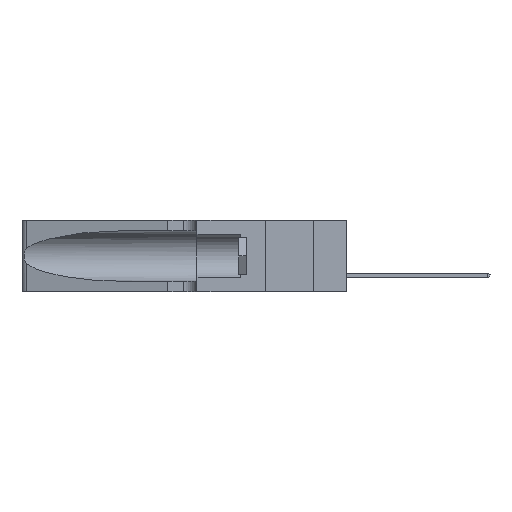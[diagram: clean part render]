
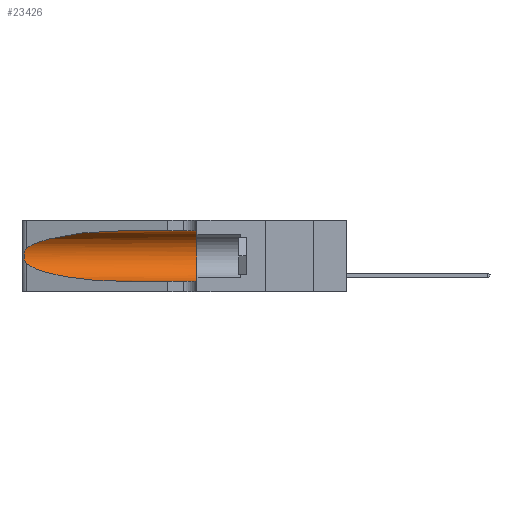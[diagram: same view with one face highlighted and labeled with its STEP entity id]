
A CAD part, left-side view. The second image highlights one B-rep face of the part: STEP entity #23426.
In plain terms, the highlighted cylindrical face has radius 3.308 mm (diameter 6.617 mm), a partial arc.
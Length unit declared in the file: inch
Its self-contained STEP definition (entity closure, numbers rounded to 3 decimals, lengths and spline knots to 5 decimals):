
#1093 = CARTESIAN_POINT ( 'NONE',  ( 0.25639, 1.23184, 0.21858 ) ) ;
#1326 = ORIENTED_EDGE ( 'NONE', *, *, #24503, .F. ) ;
#1364 = CARTESIAN_POINT ( 'NONE',  ( 0.25555, 1.22993, 0.14849 ) ) ;
#1532 = CARTESIAN_POINT ( 'NONE',  ( 0.25487, 1.22718, 0.14631 ) ) ;
#1746 = VECTOR ( 'NONE', #34111, 39.37008 ) ;
#1956 = CARTESIAN_POINT ( 'NONE',  ( 0.18966, 0.96281, 0.05475 ) ) ;
#2602 = CARTESIAN_POINT ( 'NONE',  ( 0.25487, 1.22718, 0.22369 ) ) ;
#3010 = ORIENTED_EDGE ( 'NONE', *, *, #10201, .T. ) ;
#3839 = CARTESIAN_POINT ( 'NONE',  ( 0.25854, 1.2359, 0.20912 ) ) ;
#4182 = ORIENTED_EDGE ( 'NONE', *, *, #31399, .T. ) ;
#5484 = CARTESIAN_POINT ( 'NONE',  ( 0.1305, 0.72297, 0.05475 ) ) ;
#6880 = VERTEX_POINT ( 'NONE', #2602 ) ;
#6938 = ORIENTED_EDGE ( 'NONE', *, *, #25981, .T. ) ;
#6971 = CARTESIAN_POINT ( 'NONE',  ( 0.25789, 1.23486, 0.15765 ) ) ;
#7225 = CARTESIAN_POINT ( 'NONE',  ( 0.26075, 1.23896, 0.178 ) ) ;
#7509 = CARTESIAN_POINT ( 'NONE',  ( 0.1305, 1.61858, 0.185 ) ) ;
#8089 = CIRCLE ( 'NONE', #18900, 0.13025 ) ;
#9688 = CARTESIAN_POINT ( 'NONE',  ( 0.18966, 0.96281, 0.31525 ) ) ;
#10201 = EDGE_CURVE ( 'NONE', #22672, #24491, #25761, .T. ) ;
#10582 = DIRECTION ( 'NONE',  ( 0., -1., 0. ) ) ;
#10909 = CARTESIAN_POINT ( 'NONE',  ( 0.1305, 1.61858, 0.31525 ) ) ;
#12730 = CARTESIAN_POINT ( 'NONE',  ( 0.25856, 1.23593, 0.16098 ) ) ;
#12855 = CARTESIAN_POINT ( 'NONE',  ( 0.25487, 1.22718, 0.22369 ) ) ;
#13667 = DIRECTION ( 'NONE',  ( 0., 0., -1. ) ) ;
#14142 = FACE_OUTER_BOUND ( 'NONE', #27985, .T. ) ;
#15174 = CARTESIAN_POINT ( 'NONE',  ( 0.1305, 1.61858, 0.05475 ) ) ;
#15596 = DIRECTION ( 'NONE',  ( 0., 1., 0. ) ) ;
#15795 = CARTESIAN_POINT ( 'NONE',  ( 0.25487, 1.22718, 0.14631 ) ) ;
#15982 = DIRECTION ( 'NONE',  ( 0., 0., 1. ) ) ;
#16223 = ORIENTED_EDGE ( 'NONE', *, *, #31005, .T. ) ;
#17712 = CARTESIAN_POINT ( 'NONE',  ( 0.1305, 0.72297, 0.05475 ) ) ;
#17826 = EDGE_CURVE ( 'NONE', #21288, #20216, #31760, .T. ) ;
#18103 = DIRECTION ( 'NONE',  ( 0., -1., 0. ) ) ;
#18900 = AXIS2_PLACEMENT_3D ( 'NONE', #33681, #15596, #15982 ) ;
#19483 = ORIENTED_EDGE ( 'NONE', *, *, #17826, .F. ) ;
#20050 = CARTESIAN_POINT ( 'NONE',  ( 0.1305, 0.35, 0.31525 ) ) ;
#20216 = VERTEX_POINT ( 'NONE', #20050 ) ;
#21013 = CARTESIAN_POINT ( 'NONE',  ( 0.1305, 0.72297, 0.31525 ) ) ;
#21127 = CARTESIAN_POINT ( 'NONE',  ( 0.25487, 1.22718, 0.22369 ) ) ;
#21288 = VERTEX_POINT ( 'NONE', #33509 ) ;
#22672 = VERTEX_POINT ( 'NONE', #17712 ) ;
#22736 = CARTESIAN_POINT ( 'NONE',  ( 0.2373, 1.15595, 0.08982 ) ) ;
#22876 = VERTEX_POINT ( 'NONE', #1532 ) ;
#23426 = ADVANCED_FACE ( 'NONE', ( #14142 ), #28499, .F. ) ;
#24485 = CARTESIAN_POINT ( 'NONE',  ( 0.25555, 1.22994, 0.2215 ) ) ;
#24491 = VERTEX_POINT ( 'NONE', #33408 ) ;
#24503 = EDGE_CURVE ( 'NONE', #20216, #24491, #8089, .T. ) ;
#25761 = LINE ( 'NONE', #15174, #37788 ) ;
#25981 = EDGE_CURVE ( 'NONE', #21288, #6880, #32494, .T. ) ;
#26233 = AXIS2_PLACEMENT_3D ( 'NONE', #7509, #10582, #13667 ) ;
#27466 = CARTESIAN_POINT ( 'NONE',  ( 0.25639, 1.23186, 0.15144 ) ) ;
#27984 = CARTESIAN_POINT ( 'NONE',  ( 0.25787, 1.23484, 0.2124 ) ) ;
#27985 = EDGE_LOOP ( 'NONE', ( #6938, #4182, #16223, #3010, #1326, #19483 ) ) ;
#28499 = CYLINDRICAL_SURFACE ( 'NONE', #26233, 0.13025 ) ;
#29802 = CARTESIAN_POINT ( 'NONE',  ( 0.2373, 1.15595, 0.28018 ) ) ;
#31005 = EDGE_CURVE ( 'NONE', #22876, #22672, #34169, .T. ) ;
#31399 = EDGE_CURVE ( 'NONE', #6880, #22876, #37011, .T. ) ;
#31760 = LINE ( 'NONE', #10909, #1746 ) ;
#32494 =( BOUNDED_CURVE ( )  B_SPLINE_CURVE ( 3, ( #21013, #9688, #29802, #21127 ),
 .UNSPECIFIED., .F., .T. ) 
 B_SPLINE_CURVE_WITH_KNOTS ( ( 4, 4 ),
 ( 1.5708, 2.84003 ),
 .UNSPECIFIED. ) 
 CURVE ( )  GEOMETRIC_REPRESENTATION_ITEM ( )  RATIONAL_B_SPLINE_CURVE ( ( 1., 0.87, 0.87, 1. ) ) 
 REPRESENTATION_ITEM ( '' )  );
#33408 = CARTESIAN_POINT ( 'NONE',  ( 0.1305, 0.35, 0.05475 ) ) ;
#33486 = CARTESIAN_POINT ( 'NONE',  ( 0.26018, 1.23835, 0.19895 ) ) ;
#33509 = CARTESIAN_POINT ( 'NONE',  ( 0.1305, 0.72297, 0.31525 ) ) ;
#33623 = CARTESIAN_POINT ( 'NONE',  ( 0.26075, 1.23896, 0.19203 ) ) ;
#33681 = CARTESIAN_POINT ( 'NONE',  ( 0.1305, 0.35, 0.185 ) ) ;
#34111 = DIRECTION ( 'NONE',  ( 0., -1., 0. ) ) ;
#34169 =( BOUNDED_CURVE ( )  B_SPLINE_CURVE ( 3, ( #37484, #22736, #1956, #5484 ),
 .UNSPECIFIED., .F., .F. ) 
 B_SPLINE_CURVE_WITH_KNOTS ( ( 4, 4 ),
 ( 3.44316, 4.71239 ),
 .UNSPECIFIED. ) 
 CURVE ( )  GEOMETRIC_REPRESENTATION_ITEM ( )  RATIONAL_B_SPLINE_CURVE ( ( 1., 0.87, 0.87, 1. ) ) 
 REPRESENTATION_ITEM ( '' )  );
#36760 = CARTESIAN_POINT ( 'NONE',  ( 0.26017, 1.23833, 0.17102 ) ) ;
#37011 = B_SPLINE_CURVE_WITH_KNOTS ( 'NONE', 3,
 ( #12855, #24485, #1093, #27984, #3839, #33486, #33623, #7225, #36760, #12730, #6971, #27466, #1364, #15795 ),
 .UNSPECIFIED., .F., .F.,
 ( 4, 2, 2, 2, 2, 2, 4 ),
 ( 0., 0.00027, 0.00053, 0.00107, 0.0016, 0.00187, 0.00214 ),
 .UNSPECIFIED. ) ;
#37484 = CARTESIAN_POINT ( 'NONE',  ( 0.25487, 1.22718, 0.14631 ) ) ;
#37788 = VECTOR ( 'NONE', #18103, 39.37008 ) ;
